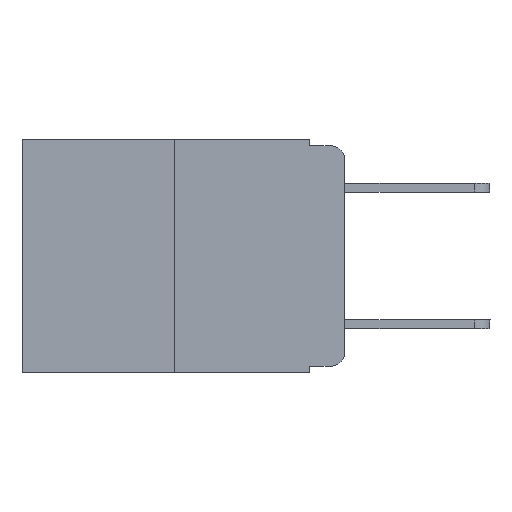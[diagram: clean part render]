
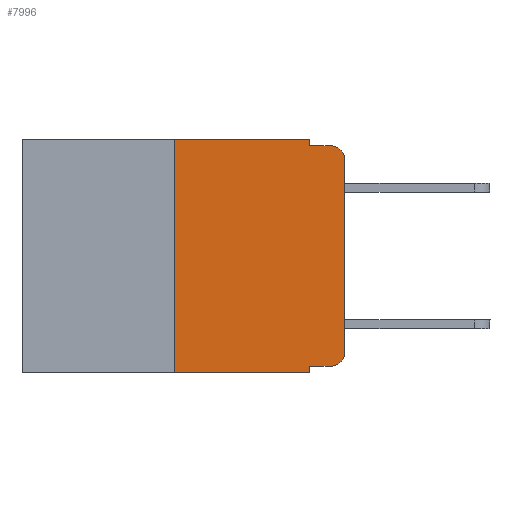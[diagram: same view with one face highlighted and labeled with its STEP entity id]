
A CAD part, left-side view. The second image highlights one B-rep face of the part: STEP entity #7996.
In plain terms, the highlighted planar face has unit normal (-1, 0, 0).
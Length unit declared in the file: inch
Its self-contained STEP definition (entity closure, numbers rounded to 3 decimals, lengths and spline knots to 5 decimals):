
#420 = AXIS2_PLACEMENT_3D ( 'NONE', #1948, #15282, #8113 ) ;
#488 = VECTOR ( 'NONE', #1811, 39.37008 ) ;
#611 = VERTEX_POINT ( 'NONE', #7432 ) ;
#698 = EDGE_CURVE ( 'NONE', #10436, #8528, #13450, .T. ) ;
#1096 = ORIENTED_EDGE ( 'NONE', *, *, #10528, .F. ) ;
#1347 = LINE ( 'NONE', #15269, #13556 ) ;
#1517 = LINE ( 'NONE', #12374, #4333 ) ;
#1731 = EDGE_CURVE ( 'NONE', #4947, #611, #9134, .T. ) ;
#1811 = DIRECTION ( 'NONE',  ( 0., 0., 1. ) ) ;
#1815 = ORIENTED_EDGE ( 'NONE', *, *, #698, .F. ) ;
#1820 = VERTEX_POINT ( 'NONE', #6517 ) ;
#1948 = CARTESIAN_POINT ( 'NONE',  ( 0., 0.02, -0.313 ) ) ;
#2086 = LINE ( 'NONE', #13435, #6780 ) ;
#2088 = DIRECTION ( 'NONE',  ( 0., -1., 0. ) ) ;
#2248 = CARTESIAN_POINT ( 'NONE',  ( 0., 0.051, 0. ) ) ;
#2798 = AXIS2_PLACEMENT_3D ( 'NONE', #4421, #6655, #13937 ) ;
#2894 = ORIENTED_EDGE ( 'NONE', *, *, #7105, .F. ) ;
#4024 = CARTESIAN_POINT ( 'NONE',  ( 0., 0.25, -0.343 ) ) ;
#4037 = VECTOR ( 'NONE', #11454, 39.37008 ) ;
#4254 = CARTESIAN_POINT ( 'NONE',  ( 0., 0.051, 0. ) ) ;
#4333 = VECTOR ( 'NONE', #11258, 39.37008 ) ;
#4421 = CARTESIAN_POINT ( 'NONE',  ( 0., 0.02, -0.03 ) ) ;
#4699 = CARTESIAN_POINT ( 'NONE',  ( 0., 0.051, -0.01 ) ) ;
#4749 = CIRCLE ( 'NONE', #420, 0.02 ) ;
#4947 = VERTEX_POINT ( 'NONE', #10482 ) ;
#5028 = VECTOR ( 'NONE', #6805, 39.37008 ) ;
#5058 = CARTESIAN_POINT ( 'NONE',  ( 0., 0.051, -0.333 ) ) ;
#5136 = DIRECTION ( 'NONE',  ( 0., 0., 1. ) ) ;
#5345 = VECTOR ( 'NONE', #8281, 39.37008 ) ;
#5407 = VERTEX_POINT ( 'NONE', #10359 ) ;
#5569 = CARTESIAN_POINT ( 'NONE',  ( 0., 0.25, 0. ) ) ;
#5660 = VERTEX_POINT ( 'NONE', #4024 ) ;
#5753 = PLANE ( 'NONE',  #12729 ) ;
#6300 = CARTESIAN_POINT ( 'NONE',  ( 0., 0.051, -0.01 ) ) ;
#6517 = CARTESIAN_POINT ( 'NONE',  ( 0., 0.02, -0.01 ) ) ;
#6655 = DIRECTION ( 'NONE',  ( -1., 0., 0. ) ) ;
#6780 = VECTOR ( 'NONE', #5136, 39.37008 ) ;
#6783 = DIRECTION ( 'NONE',  ( 1., 0., 0. ) ) ;
#6805 = DIRECTION ( 'NONE',  ( 0., 0., -1. ) ) ;
#7105 = EDGE_CURVE ( 'NONE', #5660, #10436, #2086, .T. ) ;
#7432 = CARTESIAN_POINT ( 'NONE',  ( 0., 0., -0.03 ) ) ;
#7996 = ADVANCED_FACE ( 'NONE', ( #9982 ), #5753, .F. ) ;
#8099 = ORIENTED_EDGE ( 'NONE', *, *, #1731, .T. ) ;
#8113 = DIRECTION ( 'NONE',  ( 0., 0., -1. ) ) ;
#8120 = EDGE_CURVE ( 'NONE', #8528, #14430, #15420, .T. ) ;
#8178 = DIRECTION ( 'NONE',  ( 0., 0., -1. ) ) ;
#8281 = DIRECTION ( 'NONE',  ( 0., -1., 0. ) ) ;
#8528 = VERTEX_POINT ( 'NONE', #4254 ) ;
#8777 = ORIENTED_EDGE ( 'NONE', *, *, #11712, .F. ) ;
#9003 = ORIENTED_EDGE ( 'NONE', *, *, #12836, .T. ) ;
#9134 = LINE ( 'NONE', #10035, #488 ) ;
#9472 = CIRCLE ( 'NONE', #2798, 0.02 ) ;
#9781 = ORIENTED_EDGE ( 'NONE', *, *, #12859, .T. ) ;
#9982 = FACE_OUTER_BOUND ( 'NONE', #13267, .T. ) ;
#10035 = CARTESIAN_POINT ( 'NONE',  ( 0., 0., 0. ) ) ;
#10303 = ORIENTED_EDGE ( 'NONE', *, *, #8120, .F. ) ;
#10359 = CARTESIAN_POINT ( 'NONE',  ( 0., 0.02, -0.333 ) ) ;
#10436 = VERTEX_POINT ( 'NONE', #5569 ) ;
#10482 = CARTESIAN_POINT ( 'NONE',  ( 0., 0., -0.313 ) ) ;
#10528 = EDGE_CURVE ( 'NONE', #14410, #14018, #13202, .T. ) ;
#10581 = VECTOR ( 'NONE', #15452, 39.37008 ) ;
#11258 = DIRECTION ( 'NONE',  ( 0., -1., 0. ) ) ;
#11454 = DIRECTION ( 'NONE',  ( 0., -1., 0. ) ) ;
#11712 = EDGE_CURVE ( 'NONE', #14430, #1820, #11748, .T. ) ;
#11748 = LINE ( 'NONE', #4699, #5345 ) ;
#11957 = CARTESIAN_POINT ( 'NONE',  ( 0., 0.051, 0. ) ) ;
#12077 = ORIENTED_EDGE ( 'NONE', *, *, #13726, .T. ) ;
#12374 = CARTESIAN_POINT ( 'NONE',  ( 0., 0.051, -0.333 ) ) ;
#12662 = CARTESIAN_POINT ( 'NONE',  ( 0., 0.473, 0. ) ) ;
#12729 = AXIS2_PLACEMENT_3D ( 'NONE', #14160, #6783, #8178 ) ;
#12836 = EDGE_CURVE ( 'NONE', #5407, #4947, #4749, .T. ) ;
#12859 = EDGE_CURVE ( 'NONE', #611, #1820, #9472, .T. ) ;
#13202 = LINE ( 'NONE', #2248, #5028 ) ;
#13267 = EDGE_LOOP ( 'NONE', ( #8099, #9781, #8777, #10303, #1815, #2894, #13437, #1096, #12077, #9003 ) ) ;
#13435 = CARTESIAN_POINT ( 'NONE',  ( 0., 0.25, 0. ) ) ;
#13437 = ORIENTED_EDGE ( 'NONE', *, *, #13446, .T. ) ;
#13446 = EDGE_CURVE ( 'NONE', #5660, #14018, #1347, .T. ) ;
#13450 = LINE ( 'NONE', #12662, #4037 ) ;
#13556 = VECTOR ( 'NONE', #2088, 39.37008 ) ;
#13726 = EDGE_CURVE ( 'NONE', #14410, #5407, #1517, .T. ) ;
#13937 = DIRECTION ( 'NONE',  ( 0., 0., -1. ) ) ;
#14018 = VERTEX_POINT ( 'NONE', #14167 ) ;
#14160 = CARTESIAN_POINT ( 'NONE',  ( 0., 0.473, 0. ) ) ;
#14167 = CARTESIAN_POINT ( 'NONE',  ( 0., 0.051, -0.343 ) ) ;
#14410 = VERTEX_POINT ( 'NONE', #5058 ) ;
#14430 = VERTEX_POINT ( 'NONE', #6300 ) ;
#15269 = CARTESIAN_POINT ( 'NONE',  ( 0., 0.473, -0.343 ) ) ;
#15282 = DIRECTION ( 'NONE',  ( -1., 0., 0. ) ) ;
#15420 = LINE ( 'NONE', #11957, #10581 ) ;
#15452 = DIRECTION ( 'NONE',  ( 0., 0., -1. ) ) ;
